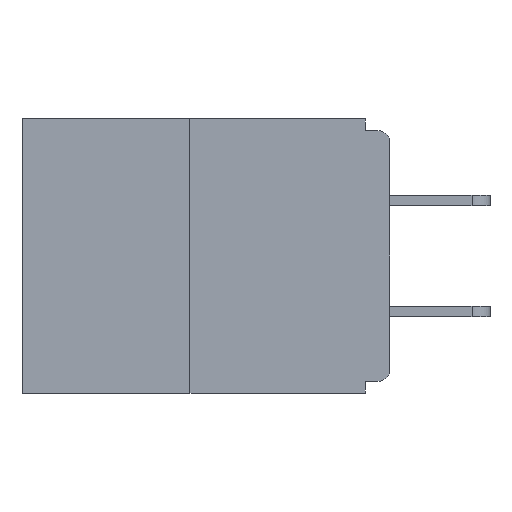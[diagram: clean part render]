
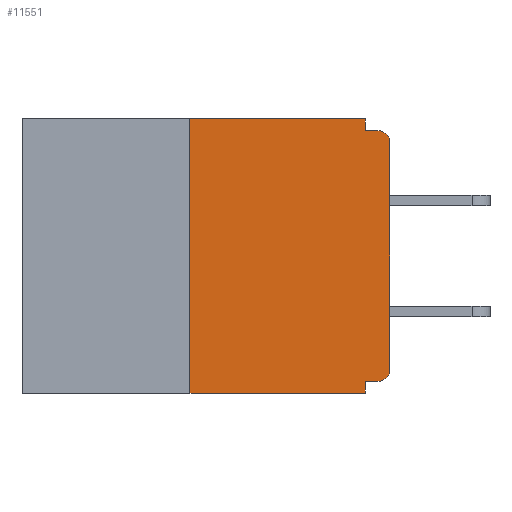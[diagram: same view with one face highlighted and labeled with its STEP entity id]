
A CAD part, left-side view. The second image highlights one B-rep face of the part: STEP entity #11551.
In plain terms, the highlighted planar face has unit normal (-1, 0, 0).
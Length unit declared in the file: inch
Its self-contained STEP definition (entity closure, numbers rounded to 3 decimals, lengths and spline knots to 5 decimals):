
#105 = EDGE_CURVE ( 'NONE', #22209, #9998, #12989, .T. ) ;
#184 = ORIENTED_EDGE ( 'NONE', *, *, #12309, .F. ) ;
#283 = CARTESIAN_POINT ( 'NONE',  ( 0., 0., 0. ) ) ;
#391 = EDGE_LOOP ( 'NONE', ( #9311, #8738, #885, #13978, #184, #8826, #19673, #4973, #7294, #8916 ) ) ;
#527 = VERTEX_POINT ( 'NONE', #6918 ) ;
#821 = FACE_OUTER_BOUND ( 'NONE', #391, .T. ) ;
#885 = ORIENTED_EDGE ( 'NONE', *, *, #14656, .T. ) ;
#1041 = EDGE_CURVE ( 'NONE', #13192, #527, #15169, .T. ) ;
#1048 = VECTOR ( 'NONE', #12034, 39.37008 ) ;
#1185 = VECTOR ( 'NONE', #6983, 39.37008 ) ;
#1657 = CARTESIAN_POINT ( 'NONE',  ( 0., 0.031, -0.015 ) ) ;
#2324 = DIRECTION ( 'NONE',  ( -1., 0., 0. ) ) ;
#2557 = EDGE_CURVE ( 'NONE', #5469, #15885, #13585, .T. ) ;
#2890 = AXIS2_PLACEMENT_3D ( 'NONE', #13683, #2324, #4698 ) ;
#3347 = DIRECTION ( 'NONE',  ( 0., 0., -1. ) ) ;
#3458 = VERTEX_POINT ( 'NONE', #11058 ) ;
#4598 = EDGE_CURVE ( 'NONE', #15885, #6755, #9294, .T. ) ;
#4698 = DIRECTION ( 'NONE',  ( 0., 0., -1. ) ) ;
#4973 = ORIENTED_EDGE ( 'NONE', *, *, #8518, .T. ) ;
#5469 = VERTEX_POINT ( 'NONE', #6499 ) ;
#5797 = LINE ( 'NONE', #23506, #1048 ) ;
#6499 = CARTESIAN_POINT ( 'NONE',  ( 0., 0.015, -0.328 ) ) ;
#6726 = AXIS2_PLACEMENT_3D ( 'NONE', #19620, #21541, #15475 ) ;
#6755 = VERTEX_POINT ( 'NONE', #12584 ) ;
#6826 = EDGE_CURVE ( 'NONE', #3458, #14872, #5797, .T. ) ;
#6918 = CARTESIAN_POINT ( 'NONE',  ( 0., 0.031, -0.343 ) ) ;
#6983 = DIRECTION ( 'NONE',  ( 0., 0., -1. ) ) ;
#7221 = CARTESIAN_POINT ( 'NONE',  ( 0., 0.25, 0. ) ) ;
#7294 = ORIENTED_EDGE ( 'NONE', *, *, #105, .F. ) ;
#7317 = DIRECTION ( 'NONE',  ( 0., 1., 0. ) ) ;
#7683 = DIRECTION ( 'NONE',  ( 0., -1., 0. ) ) ;
#8123 = VECTOR ( 'NONE', #15459, 39.37008 ) ;
#8436 = EDGE_CURVE ( 'NONE', #21994, #22209, #15815, .T. ) ;
#8518 = EDGE_CURVE ( 'NONE', #6755, #9998, #14938, .T. ) ;
#8738 = ORIENTED_EDGE ( 'NONE', *, *, #6826, .F. ) ;
#8826 = ORIENTED_EDGE ( 'NONE', *, *, #2557, .T. ) ;
#8916 = ORIENTED_EDGE ( 'NONE', *, *, #8436, .F. ) ;
#8933 = LINE ( 'NONE', #16579, #20254 ) ;
#9294 = LINE ( 'NONE', #283, #8123 ) ;
#9311 = ORIENTED_EDGE ( 'NONE', *, *, #18291, .F. ) ;
#9442 = VECTOR ( 'NONE', #7683, 39.37008 ) ;
#9948 = AXIS2_PLACEMENT_3D ( 'NONE', #11016, #20722, #3347 ) ;
#9998 = VERTEX_POINT ( 'NONE', #24130 ) ;
#10167 = CARTESIAN_POINT ( 'NONE',  ( 0., 0.031, -0.328 ) ) ;
#11016 = CARTESIAN_POINT ( 'NONE',  ( 0., 0.015, -0.03 ) ) ;
#11058 = CARTESIAN_POINT ( 'NONE',  ( 0., 0.25, -0.343 ) ) ;
#11551 = ADVANCED_FACE ( 'NONE', ( #821 ), #15642, .F. ) ;
#11755 = VECTOR ( 'NONE', #14676, 39.37008 ) ;
#12034 = DIRECTION ( 'NONE',  ( 0., 0., 1. ) ) ;
#12309 = EDGE_CURVE ( 'NONE', #5469, #13192, #14744, .T. ) ;
#12328 = DIRECTION ( 'NONE',  ( 0., 0., -1. ) ) ;
#12468 = CARTESIAN_POINT ( 'NONE',  ( 0., 0., -0.313 ) ) ;
#12584 = CARTESIAN_POINT ( 'NONE',  ( 0., 0., -0.03 ) ) ;
#12989 = LINE ( 'NONE', #14510, #11755 ) ;
#13192 = VERTEX_POINT ( 'NONE', #10167 ) ;
#13585 = CIRCLE ( 'NONE', #2890, 0.015 ) ;
#13683 = CARTESIAN_POINT ( 'NONE',  ( 0., 0.015, -0.313 ) ) ;
#13740 = CARTESIAN_POINT ( 'NONE',  ( 0., 0.46, -0.343 ) ) ;
#13978 = ORIENTED_EDGE ( 'NONE', *, *, #1041, .F. ) ;
#14510 = CARTESIAN_POINT ( 'NONE',  ( 0., 0., -0.015 ) ) ;
#14656 = EDGE_CURVE ( 'NONE', #3458, #527, #21665, .T. ) ;
#14676 = DIRECTION ( 'NONE',  ( 0., -1., 0. ) ) ;
#14744 = LINE ( 'NONE', #22752, #21595 ) ;
#14872 = VERTEX_POINT ( 'NONE', #7221 ) ;
#14938 = CIRCLE ( 'NONE', #9948, 0.015 ) ;
#15169 = LINE ( 'NONE', #23814, #1185 ) ;
#15459 = DIRECTION ( 'NONE',  ( 0., 0., 1. ) ) ;
#15475 = DIRECTION ( 'NONE',  ( 0., 0., -1. ) ) ;
#15642 = PLANE ( 'NONE',  #6726 ) ;
#15815 = LINE ( 'NONE', #23967, #17606 ) ;
#15885 = VERTEX_POINT ( 'NONE', #12468 ) ;
#16579 = CARTESIAN_POINT ( 'NONE',  ( 0., 0.46, 0. ) ) ;
#17606 = VECTOR ( 'NONE', #12328, 39.37008 ) ;
#17991 = CARTESIAN_POINT ( 'NONE',  ( 0., 0.031, 0. ) ) ;
#18291 = EDGE_CURVE ( 'NONE', #14872, #21994, #8933, .T. ) ;
#19620 = CARTESIAN_POINT ( 'NONE',  ( 0., 0.46, 0. ) ) ;
#19673 = ORIENTED_EDGE ( 'NONE', *, *, #4598, .T. ) ;
#20254 = VECTOR ( 'NONE', #23902, 39.37008 ) ;
#20722 = DIRECTION ( 'NONE',  ( -1., 0., 0. ) ) ;
#21541 = DIRECTION ( 'NONE',  ( 1., 0., 0. ) ) ;
#21595 = VECTOR ( 'NONE', #7317, 39.37008 ) ;
#21665 = LINE ( 'NONE', #13740, #9442 ) ;
#21994 = VERTEX_POINT ( 'NONE', #17991 ) ;
#22209 = VERTEX_POINT ( 'NONE', #1657 ) ;
#22752 = CARTESIAN_POINT ( 'NONE',  ( 0., 0., -0.328 ) ) ;
#23506 = CARTESIAN_POINT ( 'NONE',  ( 0., 0.25, 0. ) ) ;
#23814 = CARTESIAN_POINT ( 'NONE',  ( 0., 0.031, -0.343 ) ) ;
#23902 = DIRECTION ( 'NONE',  ( 0., -1., 0. ) ) ;
#23967 = CARTESIAN_POINT ( 'NONE',  ( 0., 0.031, 0. ) ) ;
#24130 = CARTESIAN_POINT ( 'NONE',  ( 0., 0.015, -0.015 ) ) ;
